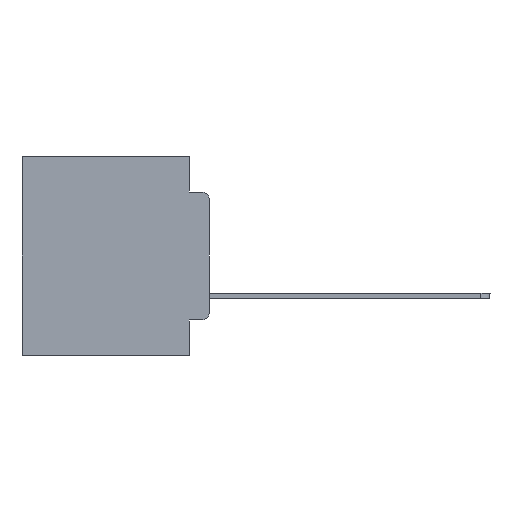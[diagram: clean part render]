
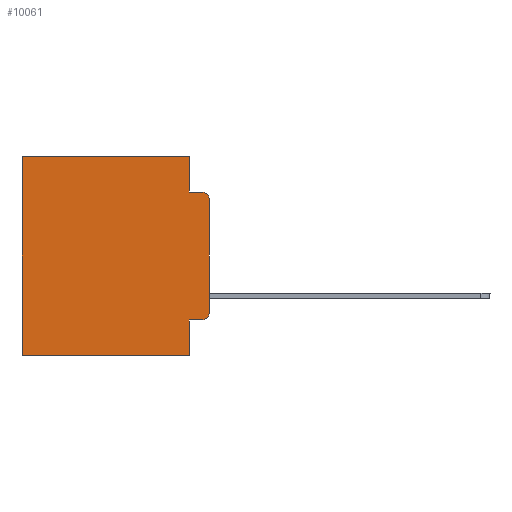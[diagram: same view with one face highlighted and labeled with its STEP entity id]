
A CAD part, left-side view. The second image highlights one B-rep face of the part: STEP entity #10061.
In plain terms, the highlighted planar face has unit normal (-1, 0, 0).
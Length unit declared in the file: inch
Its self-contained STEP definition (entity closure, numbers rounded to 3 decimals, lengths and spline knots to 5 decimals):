
#270 = EDGE_CURVE ( 'NONE', #7453, #19768, #24785, .T. ) ;
#691 = LINE ( 'NONE', #11146, #15215 ) ;
#932 = CARTESIAN_POINT ( 'NONE',  ( 0.298, 0., -0.5 ) ) ;
#974 = CARTESIAN_POINT ( 'NONE',  ( 0.298, 0.473, 0. ) ) ;
#1007 = ORIENTED_EDGE ( 'NONE', *, *, #7317, .T. ) ;
#1180 = CARTESIAN_POINT ( 'NONE',  ( 0.298, 0.051, -0.4115 ) ) ;
#1559 = CARTESIAN_POINT ( 'NONE',  ( 0.298, 0.02, -0.1085 ) ) ;
#2252 = CIRCLE ( 'NONE', #8923, 0.02 ) ;
#2442 = AXIS2_PLACEMENT_3D ( 'NONE', #8321, #6643, #15191 ) ;
#2666 = DIRECTION ( 'NONE',  ( 1., 0., 0. ) ) ;
#3554 = DIRECTION ( 'NONE',  ( 0., -1., 0. ) ) ;
#4069 = VERTEX_POINT ( 'NONE', #11906 ) ;
#4139 = VERTEX_POINT ( 'NONE', #1180 ) ;
#4384 = VECTOR ( 'NONE', #9751, 39.37008 ) ;
#4838 = VERTEX_POINT ( 'NONE', #12081 ) ;
#5861 = VERTEX_POINT ( 'NONE', #25320 ) ;
#5871 = DIRECTION ( 'NONE',  ( 0., 0., -1. ) ) ;
#6643 = DIRECTION ( 'NONE',  ( -1., 0., 0. ) ) ;
#6693 = VECTOR ( 'NONE', #17631, 39.37008 ) ;
#6795 = ORIENTED_EDGE ( 'NONE', *, *, #270, .T. ) ;
#7038 = ORIENTED_EDGE ( 'NONE', *, *, #9461, .F. ) ;
#7317 = EDGE_CURVE ( 'NONE', #7747, #5861, #9476, .T. ) ;
#7453 = VERTEX_POINT ( 'NONE', #17192 ) ;
#7626 = CARTESIAN_POINT ( 'NONE',  ( 0.298, 0.051, 0. ) ) ;
#7747 = VERTEX_POINT ( 'NONE', #7626 ) ;
#8268 = FACE_OUTER_BOUND ( 'NONE', #23527, .T. ) ;
#8321 = CARTESIAN_POINT ( 'NONE',  ( 0.298, 0.02, -0.3915 ) ) ;
#8427 = CARTESIAN_POINT ( 'NONE',  ( 0.298, 0.051, 0. ) ) ;
#8923 = AXIS2_PLACEMENT_3D ( 'NONE', #1559, #12568, #5871 ) ;
#9461 = EDGE_CURVE ( 'NONE', #24624, #4838, #27061, .T. ) ;
#9476 = LINE ( 'NONE', #26702, #4384 ) ;
#9576 = EDGE_CURVE ( 'NONE', #7747, #19757, #20755, .T. ) ;
#9751 = DIRECTION ( 'NONE',  ( 0., 1., 0. ) ) ;
#10061 = ADVANCED_FACE ( 'NONE', ( #8268 ), #16823, .F. ) ;
#10253 = CARTESIAN_POINT ( 'NONE',  ( 0.298, 0., -0.1085 ) ) ;
#11146 = CARTESIAN_POINT ( 'NONE',  ( 0.298, 0.051, -0.4115 ) ) ;
#11415 = VECTOR ( 'NONE', #16988, 39.37008 ) ;
#11906 = CARTESIAN_POINT ( 'NONE',  ( 0.298, 0.02, -0.0885 ) ) ;
#12081 = CARTESIAN_POINT ( 'NONE',  ( 0.298, 0.473, -0.5 ) ) ;
#12568 = DIRECTION ( 'NONE',  ( -1., 0., 0. ) ) ;
#13052 = EDGE_CURVE ( 'NONE', #14255, #19768, #17363, .T. ) ;
#13077 = VECTOR ( 'NONE', #16066, 39.37008 ) ;
#13146 = VECTOR ( 'NONE', #17969, 39.37008 ) ;
#13336 = EDGE_CURVE ( 'NONE', #14255, #4069, #2252, .T. ) ;
#13504 = ORIENTED_EDGE ( 'NONE', *, *, #13513, .T. ) ;
#13513 = EDGE_CURVE ( 'NONE', #4139, #7453, #691, .T. ) ;
#13781 = CARTESIAN_POINT ( 'NONE',  ( 0.298, 0.051, 0. ) ) ;
#14175 = EDGE_CURVE ( 'NONE', #4139, #24624, #24415, .T. ) ;
#14255 = VERTEX_POINT ( 'NONE', #10253 ) ;
#14279 = ORIENTED_EDGE ( 'NONE', *, *, #21384, .F. ) ;
#14679 = ORIENTED_EDGE ( 'NONE', *, *, #9576, .F. ) ;
#14791 = VECTOR ( 'NONE', #22291, 39.37008 ) ;
#15191 = DIRECTION ( 'NONE',  ( 0., 0., -1. ) ) ;
#15215 = VECTOR ( 'NONE', #21908, 39.37008 ) ;
#15802 = LINE ( 'NONE', #974, #13077 ) ;
#16066 = DIRECTION ( 'NONE',  ( 0., 0., -1. ) ) ;
#16823 = PLANE ( 'NONE',  #19066 ) ;
#16988 = DIRECTION ( 'NONE',  ( 0., 0., -1. ) ) ;
#17192 = CARTESIAN_POINT ( 'NONE',  ( 0.298, 0.02, -0.4115 ) ) ;
#17363 = LINE ( 'NONE', #21938, #6693 ) ;
#17503 = DIRECTION ( 'NONE',  ( 0., 0., -1. ) ) ;
#17631 = DIRECTION ( 'NONE',  ( 0., 0., -1. ) ) ;
#17969 = DIRECTION ( 'NONE',  ( 0., 1., 0. ) ) ;
#18371 = LINE ( 'NONE', #24823, #19866 ) ;
#18402 = CARTESIAN_POINT ( 'NONE',  ( 0.298, 0.051, -0.0885 ) ) ;
#19066 = AXIS2_PLACEMENT_3D ( 'NONE', #25340, #2666, #17503 ) ;
#19757 = VERTEX_POINT ( 'NONE', #18402 ) ;
#19768 = VERTEX_POINT ( 'NONE', #22314 ) ;
#19866 = VECTOR ( 'NONE', #3554, 39.37008 ) ;
#20755 = LINE ( 'NONE', #8427, #11415 ) ;
#20821 = ORIENTED_EDGE ( 'NONE', *, *, #25504, .T. ) ;
#21188 = ORIENTED_EDGE ( 'NONE', *, *, #13052, .F. ) ;
#21384 = EDGE_CURVE ( 'NONE', #19757, #4069, #18371, .T. ) ;
#21908 = DIRECTION ( 'NONE',  ( 0., -1., 0. ) ) ;
#21938 = CARTESIAN_POINT ( 'NONE',  ( 0.298, 0., 0. ) ) ;
#22291 = DIRECTION ( 'NONE',  ( 0., 0., -1. ) ) ;
#22314 = CARTESIAN_POINT ( 'NONE',  ( 0.298, 0., -0.3915 ) ) ;
#23527 = EDGE_LOOP ( 'NONE', ( #21188, #24797, #14279, #14679, #1007, #20821, #7038, #26001, #13504, #6795 ) ) ;
#24280 = CARTESIAN_POINT ( 'NONE',  ( 0.298, 0.051, -0.5 ) ) ;
#24415 = LINE ( 'NONE', #13781, #14791 ) ;
#24624 = VERTEX_POINT ( 'NONE', #24280 ) ;
#24785 = CIRCLE ( 'NONE', #2442, 0.02 ) ;
#24797 = ORIENTED_EDGE ( 'NONE', *, *, #13336, .T. ) ;
#24823 = CARTESIAN_POINT ( 'NONE',  ( 0.298, 0.051, -0.0885 ) ) ;
#25320 = CARTESIAN_POINT ( 'NONE',  ( 0.298, 0.473, 0. ) ) ;
#25340 = CARTESIAN_POINT ( 'NONE',  ( 0.298, 0., 0. ) ) ;
#25504 = EDGE_CURVE ( 'NONE', #5861, #4838, #15802, .T. ) ;
#26001 = ORIENTED_EDGE ( 'NONE', *, *, #14175, .F. ) ;
#26702 = CARTESIAN_POINT ( 'NONE',  ( 0.298, 0., 0. ) ) ;
#27061 = LINE ( 'NONE', #932, #13146 ) ;
